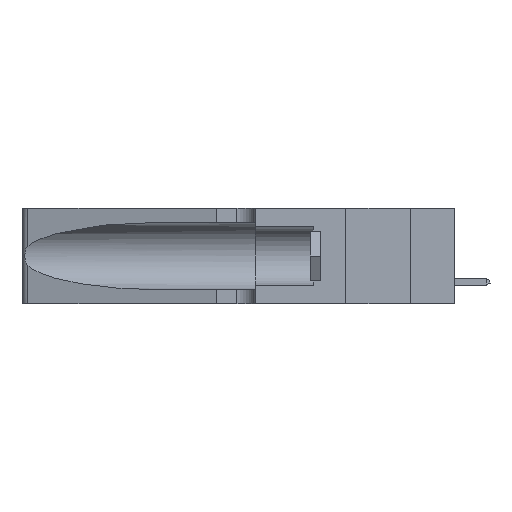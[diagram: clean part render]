
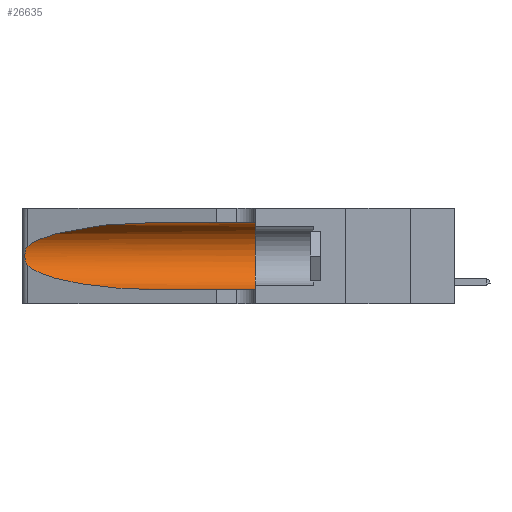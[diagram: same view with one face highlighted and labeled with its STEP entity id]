
A CAD part, left-side view. The second image highlights one B-rep face of the part: STEP entity #26635.
In plain terms, the highlighted cylindrical face has radius 3.308 mm (diameter 6.617 mm), a partial arc.
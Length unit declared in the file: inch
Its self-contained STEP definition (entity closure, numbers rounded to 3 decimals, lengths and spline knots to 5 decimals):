
#58 = EDGE_CURVE ( 'NONE', #31227, #12465, #10226, .T. ) ;
#2027 = DIRECTION ( 'NONE',  ( 0., -1., 0. ) ) ;
#2040 = VERTEX_POINT ( 'NONE', #30639 ) ;
#2044 = EDGE_CURVE ( 'NONE', #2040, #12465, #22757, .T. ) ;
#2187 = FACE_OUTER_BOUND ( 'NONE', #30490, .T. ) ;
#2523 = CARTESIAN_POINT ( 'NONE',  ( 0.25639, 1.23184, 0.21858 ) ) ;
#2607 = DIRECTION ( 'NONE',  ( 0., -1., 0. ) ) ;
#2836 = CARTESIAN_POINT ( 'NONE',  ( 0.26075, 1.23896, 0.178 ) ) ;
#3877 = CARTESIAN_POINT ( 'NONE',  ( 0.25487, 1.22718, 0.22369 ) ) ;
#4291 = CARTESIAN_POINT ( 'NONE',  ( 0.18966, 0.96281, 0.31525 ) ) ;
#4826 = CARTESIAN_POINT ( 'NONE',  ( 0.2373, 1.15595, 0.08982 ) ) ;
#4951 = LINE ( 'NONE', #6739, #19585 ) ;
#5026 = CARTESIAN_POINT ( 'NONE',  ( 0.26075, 1.23896, 0.19203 ) ) ;
#6739 = CARTESIAN_POINT ( 'NONE',  ( 0.1305, 1.61858, 0.31525 ) ) ;
#7248 = ORIENTED_EDGE ( 'NONE', *, *, #17408, .F. ) ;
#7446 = CARTESIAN_POINT ( 'NONE',  ( 0.25555, 1.22994, 0.2215 ) ) ;
#7765 = CARTESIAN_POINT ( 'NONE',  ( 0.25555, 1.22993, 0.14849 ) ) ;
#7873 = CARTESIAN_POINT ( 'NONE',  ( 0.25854, 1.2359, 0.20912 ) ) ;
#8706 = ORIENTED_EDGE ( 'NONE', *, *, #31345, .T. ) ;
#9327 = ORIENTED_EDGE ( 'NONE', *, *, #21817, .T. ) ;
#9500 = VERTEX_POINT ( 'NONE', #25653 ) ;
#10226 = CIRCLE ( 'NONE', #22830, 0.13025 ) ;
#10323 = CARTESIAN_POINT ( 'NONE',  ( 0.25789, 1.23486, 0.15765 ) ) ;
#10950 = VECTOR ( 'NONE', #12986, 39.37008 ) ;
#11134 = CARTESIAN_POINT ( 'NONE',  ( 0.1305, 0.72297, 0.31525 ) ) ;
#11452 = ORIENTED_EDGE ( 'NONE', *, *, #14907, .T. ) ;
#11461 = CARTESIAN_POINT ( 'NONE',  ( 0.1305, 0.35, 0.31525 ) ) ;
#12465 = VERTEX_POINT ( 'NONE', #20767 ) ;
#12536 =( BOUNDED_CURVE ( )  B_SPLINE_CURVE ( 3, ( #19721, #4826, #14764, #22161 ),
 .UNSPECIFIED., .F., .F. ) 
 B_SPLINE_CURVE_WITH_KNOTS ( ( 4, 4 ),
 ( 3.44316, 4.71239 ),
 .UNSPECIFIED. ) 
 CURVE ( )  GEOMETRIC_REPRESENTATION_ITEM ( )  RATIONAL_B_SPLINE_CURVE ( ( 1., 0.87, 0.87, 1. ) ) 
 REPRESENTATION_ITEM ( '' )  );
#12741 = CARTESIAN_POINT ( 'NONE',  ( 0.26017, 1.23833, 0.17102 ) ) ;
#12986 = DIRECTION ( 'NONE',  ( 0., -1., 0. ) ) ;
#13674 = VERTEX_POINT ( 'NONE', #11134 ) ;
#14170 = ORIENTED_EDGE ( 'NONE', *, *, #58, .F. ) ;
#14415 = CYLINDRICAL_SURFACE ( 'NONE', #28452, 0.13025 ) ;
#14731 = VERTEX_POINT ( 'NONE', #21161 ) ;
#14764 = CARTESIAN_POINT ( 'NONE',  ( 0.18966, 0.96281, 0.05475 ) ) ;
#14907 = EDGE_CURVE ( 'NONE', #13674, #14731, #20851, .T. ) ;
#15403 = CARTESIAN_POINT ( 'NONE',  ( 0.26018, 1.23835, 0.19895 ) ) ;
#17408 = EDGE_CURVE ( 'NONE', #13674, #31227, #4951, .T. ) ;
#18521 = CARTESIAN_POINT ( 'NONE',  ( 0.1305, 0.72297, 0.31525 ) ) ;
#19585 = VECTOR ( 'NONE', #2027, 39.37008 ) ;
#19721 = CARTESIAN_POINT ( 'NONE',  ( 0.25487, 1.22718, 0.14631 ) ) ;
#20033 = CARTESIAN_POINT ( 'NONE',  ( 0.25487, 1.22718, 0.22369 ) ) ;
#20135 = CARTESIAN_POINT ( 'NONE',  ( 0.25787, 1.23484, 0.2124 ) ) ;
#20243 = CARTESIAN_POINT ( 'NONE',  ( 0.25856, 1.23593, 0.16098 ) ) ;
#20767 = CARTESIAN_POINT ( 'NONE',  ( 0.1305, 0.35, 0.05475 ) ) ;
#20851 =( BOUNDED_CURVE ( )  B_SPLINE_CURVE ( 3, ( #18521, #4291, #31764, #3877 ),
 .UNSPECIFIED., .F., .F. ) 
 B_SPLINE_CURVE_WITH_KNOTS ( ( 4, 4 ),
 ( 1.5708, 2.84003 ),
 .UNSPECIFIED. ) 
 CURVE ( )  GEOMETRIC_REPRESENTATION_ITEM ( )  RATIONAL_B_SPLINE_CURVE ( ( 1., 0.87, 0.87, 1. ) ) 
 REPRESENTATION_ITEM ( '' )  );
#21161 = CARTESIAN_POINT ( 'NONE',  ( 0.25487, 1.22718, 0.22369 ) ) ;
#21817 = EDGE_CURVE ( 'NONE', #14731, #9500, #31173, .T. ) ;
#21882 = DIRECTION ( 'NONE',  ( 0., 1., 0. ) ) ;
#22161 = CARTESIAN_POINT ( 'NONE',  ( 0.1305, 0.72297, 0.05475 ) ) ;
#22757 = LINE ( 'NONE', #25106, #10950 ) ;
#22830 = AXIS2_PLACEMENT_3D ( 'NONE', #32040, #21882, #29570 ) ;
#25106 = CARTESIAN_POINT ( 'NONE',  ( 0.1305, 1.61858, 0.05475 ) ) ;
#25420 = CARTESIAN_POINT ( 'NONE',  ( 0.25487, 1.22718, 0.14631 ) ) ;
#25630 = CARTESIAN_POINT ( 'NONE',  ( 0.1305, 1.61858, 0.185 ) ) ;
#25653 = CARTESIAN_POINT ( 'NONE',  ( 0.25487, 1.22718, 0.14631 ) ) ;
#26635 = ADVANCED_FACE ( 'NONE', ( #2187 ), #14415, .F. ) ;
#28139 = DIRECTION ( 'NONE',  ( 0., 0., -1. ) ) ;
#28452 = AXIS2_PLACEMENT_3D ( 'NONE', #25630, #2607, #28139 ) ;
#29570 = DIRECTION ( 'NONE',  ( 0., 0., 1. ) ) ;
#29767 = ORIENTED_EDGE ( 'NONE', *, *, #2044, .T. ) ;
#30402 = CARTESIAN_POINT ( 'NONE',  ( 0.25639, 1.23186, 0.15144 ) ) ;
#30490 = EDGE_LOOP ( 'NONE', ( #11452, #9327, #8706, #29767, #14170, #7248 ) ) ;
#30639 = CARTESIAN_POINT ( 'NONE',  ( 0.1305, 0.72297, 0.05475 ) ) ;
#31173 = B_SPLINE_CURVE_WITH_KNOTS ( 'NONE', 3,
 ( #20033, #7446, #2523, #20135, #7873, #15403, #5026, #2836, #12741, #20243, #10323, #30402, #7765, #25420 ),
 .UNSPECIFIED., .F., .F.,
 ( 4, 2, 2, 2, 2, 2, 4 ),
 ( 0., 0.00027, 0.00053, 0.00107, 0.0016, 0.00187, 0.00214 ),
 .UNSPECIFIED. ) ;
#31227 = VERTEX_POINT ( 'NONE', #11461 ) ;
#31345 = EDGE_CURVE ( 'NONE', #9500, #2040, #12536, .T. ) ;
#31764 = CARTESIAN_POINT ( 'NONE',  ( 0.2373, 1.15595, 0.28018 ) ) ;
#32040 = CARTESIAN_POINT ( 'NONE',  ( 0.1305, 0.35, 0.185 ) ) ;
